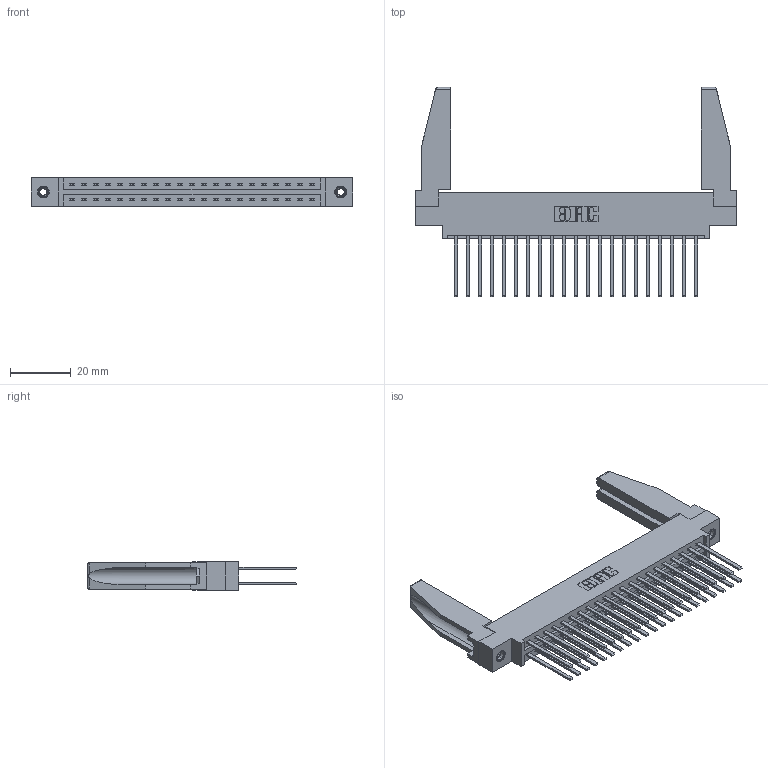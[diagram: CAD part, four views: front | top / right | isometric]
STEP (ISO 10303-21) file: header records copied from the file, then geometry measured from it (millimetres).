
FILE_DESCRIPTION (( 'STEP AP203' ), '1' );
FILE_NAME ('387-042-544-878.STEP', '2019-10-18T04:27:17', ( '' ), ( '' ), 'SwSTEP 2.0', 'SolidWorks 2016', '' );
FILE_SCHEMA (( 'CONFIG_CONTROL_DESIGN' ));
Length unit declared in the file: inch
Products named in the file (5): 345-250-001_345-250-001-102; 387-042-544-878; 345-292-001_345-293-144; 337 Part_0.170 Offset - 0.156 Dia-TI; 307-220-078
Assembly tree (47 placements, depth 2):
  387-042-544-878
    337 Part_0.170 Offset - 0.156 Dia-TI
    345-292-001_345-293-144  x42
    345-250-001_345-250-001-102  x2
    307-220-078  x2
Bounding box: 106.22 x 69.09 x 9.4 mm (x, y, z)
Volume: 15379.7 mm3; surface area: 18529.9 mm2
Topology: 47 solids, 47 shells, 2264 faces, 6659 edges, 4374 vertices
Faces by surface type: plane 1586, cylinder 662, cone 12, torus 4
Entity records: 21386 total; most frequent: CARTESIAN_POINT 3620, ORIENTED_EDGE 3512, DIRECTION 3120, EDGE_CURVE 1756, VECTOR 1594, LINE 1594, VERTEX_POINT 1164, AXIS2_PLACEMENT_3D 763
